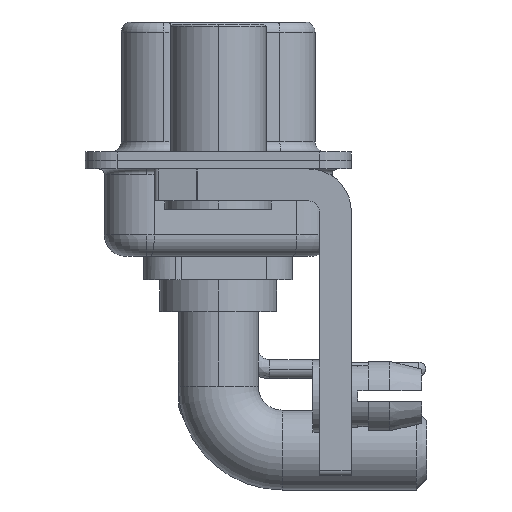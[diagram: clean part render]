
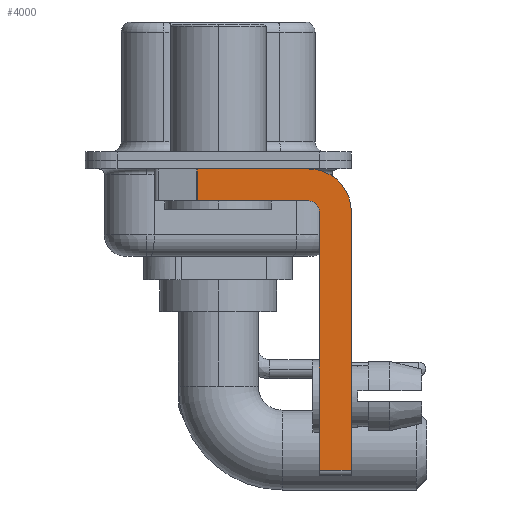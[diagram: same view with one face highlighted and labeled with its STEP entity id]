
A CAD part, left-side view. The second image highlights one B-rep face of the part: STEP entity #4000.
In plain terms, the highlighted planar face has unit normal (-1, 0, 0).
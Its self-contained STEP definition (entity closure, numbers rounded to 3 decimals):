
#1 = EDGE_CURVE ( 'NONE', #258, #17609, #3351, .T. ) ;
#164 = VERTEX_POINT ( 'NONE', #22137 ) ;
#258 = VERTEX_POINT ( 'NONE', #13491 ) ;
#548 = CARTESIAN_POINT ( 'NONE',  ( -2.9, 3., -0.4 ) ) ;
#839 = PLANE ( 'NONE',  #20989 ) ;
#1190 = VERTEX_POINT ( 'NONE', #15746 ) ;
#2246 = DIRECTION ( 'NONE',  ( 0., -1., 0. ) ) ;
#2715 = DIRECTION ( 'NONE',  ( 1., 0., 0. ) ) ;
#2984 = DIRECTION ( 'NONE',  ( 0., 0., -1. ) ) ;
#3351 = CIRCLE ( 'NONE', #24388, 2. ) ;
#3469 = DIRECTION ( 'NONE',  ( 0., 0., -1. ) ) ;
#3763 = EDGE_CURVE ( 'NONE', #1190, #164, #14574, .T. ) ;
#3962 = EDGE_CURVE ( 'NONE', #1190, #258, #16004, .T. ) ;
#4000 = ADVANCED_FACE ( 'NONE', ( #16153 ), #839, .F. ) ;
#4499 = ORIENTED_EDGE ( 'NONE', *, *, #23726, .F. ) ;
#4707 = CARTESIAN_POINT ( 'NONE',  ( -2.9, -4.25, -14.55 ) ) ;
#4839 = ORIENTED_EDGE ( 'NONE', *, *, #16201, .T. ) ;
#5471 = LINE ( 'NONE', #14373, #7113 ) ;
#5729 = CARTESIAN_POINT ( 'NONE',  ( -2.9, -4.25, -1.9 ) ) ;
#6059 = VECTOR ( 'NONE', #20706, 1000. ) ;
#6634 = LINE ( 'NONE', #4707, #25777 ) ;
#7113 = VECTOR ( 'NONE', #2984, 1000. ) ;
#7812 = EDGE_LOOP ( 'NONE', ( #27782, #23426, #12564, #4499, #13970, #4839, #19712, #18990 ) ) ;
#8176 = LINE ( 'NONE', #17066, #12075 ) ;
#9129 = VERTEX_POINT ( 'NONE', #17349 ) ;
#9746 = CARTESIAN_POINT ( 'NONE',  ( -2.9, -4.25, -2.4 ) ) ;
#10345 = EDGE_CURVE ( 'NONE', #23003, #9129, #8176, .T. ) ;
#10986 = DIRECTION ( 'NONE',  ( 1., 0., 0. ) ) ;
#12075 = VECTOR ( 'NONE', #15023, 1000. ) ;
#12564 = ORIENTED_EDGE ( 'NONE', *, *, #16311, .F. ) ;
#13200 = DIRECTION ( 'NONE',  ( 0., 1., 0. ) ) ;
#13491 = CARTESIAN_POINT ( 'NONE',  ( -2.9, -4.25, -0.4 ) ) ;
#13673 = VERTEX_POINT ( 'NONE', #5729 ) ;
#13970 = ORIENTED_EDGE ( 'NONE', *, *, #10345, .F. ) ;
#14373 = CARTESIAN_POINT ( 'NONE',  ( -2.9, -6.25, -2.4 ) ) ;
#14574 = LINE ( 'NONE', #23513, #16246 ) ;
#15023 = DIRECTION ( 'NONE',  ( 0., 0., 1. ) ) ;
#15295 = AXIS2_PLACEMENT_3D ( 'NONE', #20251, #22593, #19830 ) ;
#15746 = CARTESIAN_POINT ( 'NONE',  ( -2.9, 0.978, -0.4 ) ) ;
#15974 = EDGE_CURVE ( 'NONE', #17609, #24173, #5471, .T. ) ;
#16004 = LINE ( 'NONE', #548, #6059 ) ;
#16153 = FACE_OUTER_BOUND ( 'NONE', #7812, .T. ) ;
#16201 = EDGE_CURVE ( 'NONE', #23003, #24173, #6634, .T. ) ;
#16246 = VECTOR ( 'NONE', #3469, 1000. ) ;
#16311 = EDGE_CURVE ( 'NONE', #13673, #164, #26921, .T. ) ;
#17066 = CARTESIAN_POINT ( 'NONE',  ( -2.9, -4.75, -14.8 ) ) ;
#17349 = CARTESIAN_POINT ( 'NONE',  ( -2.9, -4.75, -2.4 ) ) ;
#17609 = VERTEX_POINT ( 'NONE', #24063 ) ;
#18990 = ORIENTED_EDGE ( 'NONE', *, *, #1, .F. ) ;
#19610 = DIRECTION ( 'NONE',  ( 0., 0., -1. ) ) ;
#19712 = ORIENTED_EDGE ( 'NONE', *, *, #15974, .F. ) ;
#19717 = VECTOR ( 'NONE', #13200, 1000. ) ;
#19830 = DIRECTION ( 'NONE',  ( 0., 0., 1. ) ) ;
#19973 = CIRCLE ( 'NONE', #15295, 0.5 ) ;
#20251 = CARTESIAN_POINT ( 'NONE',  ( -2.9, -4.25, -2.4 ) ) ;
#20706 = DIRECTION ( 'NONE',  ( 0., -1., 0. ) ) ;
#20989 = AXIS2_PLACEMENT_3D ( 'NONE', #9746, #2715, #25080 ) ;
#22137 = CARTESIAN_POINT ( 'NONE',  ( -2.9, 0.978, -1.9 ) ) ;
#22593 = DIRECTION ( 'NONE',  ( -1., 0., 0. ) ) ;
#23003 = VERTEX_POINT ( 'NONE', #25681 ) ;
#23426 = ORIENTED_EDGE ( 'NONE', *, *, #3763, .T. ) ;
#23513 = CARTESIAN_POINT ( 'NONE',  ( -2.9, 0.978, -1.9 ) ) ;
#23726 = EDGE_CURVE ( 'NONE', #9129, #13673, #19973, .T. ) ;
#24063 = CARTESIAN_POINT ( 'NONE',  ( -2.9, -6.25, -2.4 ) ) ;
#24173 = VERTEX_POINT ( 'NONE', #26791 ) ;
#24388 = AXIS2_PLACEMENT_3D ( 'NONE', #28670, #10986, #19610 ) ;
#25080 = DIRECTION ( 'NONE',  ( 0., 0., -1. ) ) ;
#25681 = CARTESIAN_POINT ( 'NONE',  ( -2.9, -4.75, -14.55 ) ) ;
#25777 = VECTOR ( 'NONE', #2246, 1000. ) ;
#26785 = CARTESIAN_POINT ( 'NONE',  ( -2.9, -4.25, -1.9 ) ) ;
#26791 = CARTESIAN_POINT ( 'NONE',  ( -2.9, -6.25, -14.55 ) ) ;
#26921 = LINE ( 'NONE', #26785, #19717 ) ;
#27782 = ORIENTED_EDGE ( 'NONE', *, *, #3962, .F. ) ;
#28670 = CARTESIAN_POINT ( 'NONE',  ( -2.9, -4.25, -2.4 ) ) ;
